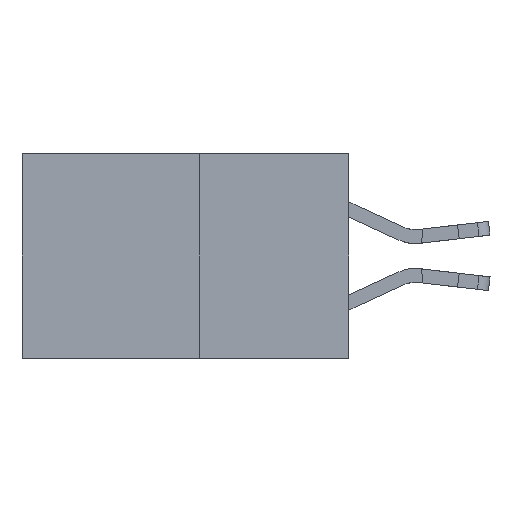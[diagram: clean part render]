
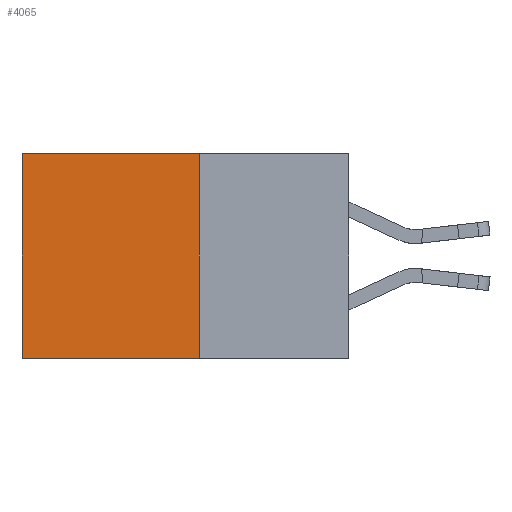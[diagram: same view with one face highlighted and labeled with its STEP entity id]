
A CAD part, left-side view. The second image highlights one B-rep face of the part: STEP entity #4065.
In plain terms, the highlighted planar face has unit normal (-1, 0, 0).
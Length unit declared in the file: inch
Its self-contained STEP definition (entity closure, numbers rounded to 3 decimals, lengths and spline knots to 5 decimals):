
#1003 = DIRECTION ( 'NONE',  ( 0., 0., -1. ) ) ;
#1072 = CARTESIAN_POINT ( 'NONE',  ( 0.277, 0.59, -0.37 ) ) ;
#1179 = LINE ( 'NONE', #19297, #17821 ) ;
#1367 = VECTOR ( 'NONE', #1003, 39.37008 ) ;
#2307 = DIRECTION ( 'NONE',  ( 0., 1., 0. ) ) ;
#2319 = DIRECTION ( 'NONE',  ( 0., 0., -1. ) ) ;
#2443 = DIRECTION ( 'NONE',  ( 1., 0., 0. ) ) ;
#2660 = CARTESIAN_POINT ( 'NONE',  ( 0.277, 0.27, -0.37 ) ) ;
#2756 = PLANE ( 'NONE',  #5894 ) ;
#2784 = VECTOR ( 'NONE', #2307, 39.37008 ) ;
#2842 = VERTEX_POINT ( 'NONE', #8394 ) ;
#3375 = DIRECTION ( 'NONE',  ( 0., 1., 0. ) ) ;
#3573 = EDGE_CURVE ( 'NONE', #17809, #2842, #19781, .T. ) ;
#4006 = CARTESIAN_POINT ( 'NONE',  ( 0.277, 0.27, -0.37 ) ) ;
#4065 = ADVANCED_FACE ( 'NONE', ( #18306 ), #2756, .F. ) ;
#4166 = VERTEX_POINT ( 'NONE', #7923 ) ;
#5894 = AXIS2_PLACEMENT_3D ( 'NONE', #2660, #2443, #2319 ) ;
#6977 = EDGE_CURVE ( 'NONE', #2842, #4166, #13779, .T. ) ;
#7217 = ORIENTED_EDGE ( 'NONE', *, *, #11783, .F. ) ;
#7923 = CARTESIAN_POINT ( 'NONE',  ( 0.277, 0.59, -0.37 ) ) ;
#8190 = ORIENTED_EDGE ( 'NONE', *, *, #3573, .T. ) ;
#8394 = CARTESIAN_POINT ( 'NONE',  ( 0.277, 0.59, 0. ) ) ;
#11012 = LINE ( 'NONE', #11888, #19890 ) ;
#11288 = ORIENTED_EDGE ( 'NONE', *, *, #6977, .T. ) ;
#11487 = DIRECTION ( 'NONE',  ( 0., 0., -1. ) ) ;
#11783 = EDGE_CURVE ( 'NONE', #17809, #18103, #11012, .T. ) ;
#11888 = CARTESIAN_POINT ( 'NONE',  ( 0.277, 0.27, -0.37 ) ) ;
#13779 = LINE ( 'NONE', #1072, #1367 ) ;
#15483 = ORIENTED_EDGE ( 'NONE', *, *, #15554, .F. ) ;
#15554 = EDGE_CURVE ( 'NONE', #18103, #4166, #1179, .T. ) ;
#16847 = CARTESIAN_POINT ( 'NONE',  ( 0.277, 0.27, 0. ) ) ;
#17809 = VERTEX_POINT ( 'NONE', #19224 ) ;
#17821 = VECTOR ( 'NONE', #3375, 39.37008 ) ;
#18103 = VERTEX_POINT ( 'NONE', #4006 ) ;
#18306 = FACE_OUTER_BOUND ( 'NONE', #19998, .T. ) ;
#19224 = CARTESIAN_POINT ( 'NONE',  ( 0.277, 0.27, 0. ) ) ;
#19297 = CARTESIAN_POINT ( 'NONE',  ( 0.277, 0.27, -0.37 ) ) ;
#19781 = LINE ( 'NONE', #16847, #2784 ) ;
#19890 = VECTOR ( 'NONE', #11487, 39.37008 ) ;
#19998 = EDGE_LOOP ( 'NONE', ( #11288, #15483, #7217, #8190 ) ) ;
